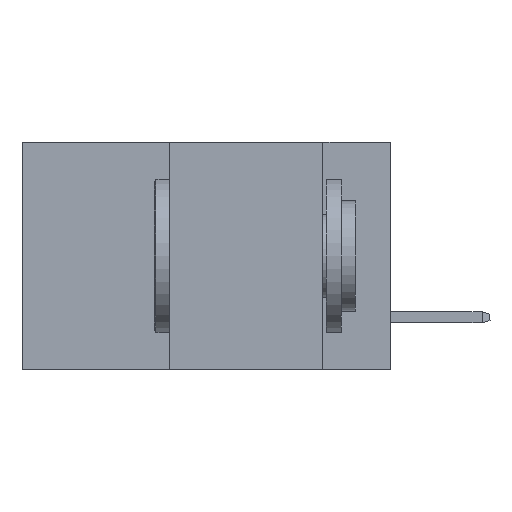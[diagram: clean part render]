
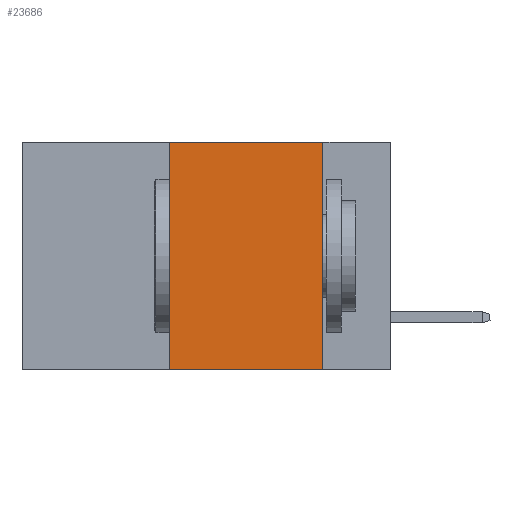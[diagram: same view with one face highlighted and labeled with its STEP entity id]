
A CAD part, left-side view. The second image highlights one B-rep face of the part: STEP entity #23686.
In plain terms, the highlighted planar face has unit normal (-1, 0, 0).
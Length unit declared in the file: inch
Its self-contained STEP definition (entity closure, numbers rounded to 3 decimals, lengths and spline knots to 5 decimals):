
#117 = ORIENTED_EDGE ( 'NONE', *, *, #20808, .F. ) ;
#3116 = ORIENTED_EDGE ( 'NONE', *, *, #18078, .T. ) ;
#3369 = DIRECTION ( 'NONE',  ( 0., 0., -1. ) ) ;
#3639 = CARTESIAN_POINT ( 'NONE',  ( 0., 0.11, 0. ) ) ;
#4023 = VECTOR ( 'NONE', #17754, 39.37008 ) ;
#4183 = EDGE_LOOP ( 'NONE', ( #18869, #117, #10741, #3116 ) ) ;
#4851 = VERTEX_POINT ( 'NONE', #25105 ) ;
#4886 = VECTOR ( 'NONE', #9809, 39.37008 ) ;
#5195 = VERTEX_POINT ( 'NONE', #3639 ) ;
#5243 = CARTESIAN_POINT ( 'NONE',  ( 0., 0.36, -0.37 ) ) ;
#5410 = LINE ( 'NONE', #6301, #26927 ) ;
#6301 = CARTESIAN_POINT ( 'NONE',  ( 0., 0.6, -0.37 ) ) ;
#6917 = CARTESIAN_POINT ( 'NONE',  ( 0., 0.36, 0. ) ) ;
#7894 = CARTESIAN_POINT ( 'NONE',  ( 0., 0.11, 0. ) ) ;
#9809 = DIRECTION ( 'NONE',  ( 0., -1., 0. ) ) ;
#9952 = LINE ( 'NONE', #6917, #4023 ) ;
#10741 = ORIENTED_EDGE ( 'NONE', *, *, #26559, .F. ) ;
#10774 = DIRECTION ( 'NONE',  ( 0., 0., -1. ) ) ;
#13309 = VERTEX_POINT ( 'NONE', #5243 ) ;
#17754 = DIRECTION ( 'NONE',  ( 0., 0., 1. ) ) ;
#18078 = EDGE_CURVE ( 'NONE', #13309, #4851, #5410, .T. ) ;
#18420 = CARTESIAN_POINT ( 'NONE',  ( 0., 0.6, 0. ) ) ;
#18869 = ORIENTED_EDGE ( 'NONE', *, *, #27935, .F. ) ;
#19965 = CARTESIAN_POINT ( 'NONE',  ( 0., 0.36, 0. ) ) ;
#20808 = EDGE_CURVE ( 'NONE', #21835, #5195, #22862, .T. ) ;
#21355 = VECTOR ( 'NONE', #3369, 39.37008 ) ;
#21484 = CARTESIAN_POINT ( 'NONE',  ( 0., 0.6, 0. ) ) ;
#21835 = VERTEX_POINT ( 'NONE', #19965 ) ;
#22037 = LINE ( 'NONE', #7894, #21355 ) ;
#22862 = LINE ( 'NONE', #18420, #4886 ) ;
#23577 = DIRECTION ( 'NONE',  ( 0., -1., 0. ) ) ;
#23650 = DIRECTION ( 'NONE',  ( 1., 0., 0. ) ) ;
#23686 = ADVANCED_FACE ( 'NONE', ( #27149 ), #27710, .F. ) ;
#25052 = AXIS2_PLACEMENT_3D ( 'NONE', #21484, #23650, #10774 ) ;
#25105 = CARTESIAN_POINT ( 'NONE',  ( 0., 0.11, -0.37 ) ) ;
#26559 = EDGE_CURVE ( 'NONE', #13309, #21835, #9952, .T. ) ;
#26927 = VECTOR ( 'NONE', #23577, 39.37008 ) ;
#27149 = FACE_OUTER_BOUND ( 'NONE', #4183, .T. ) ;
#27710 = PLANE ( 'NONE',  #25052 ) ;
#27935 = EDGE_CURVE ( 'NONE', #5195, #4851, #22037, .T. ) ;
